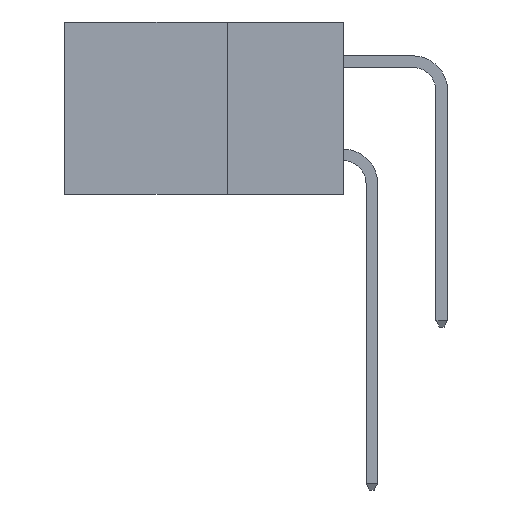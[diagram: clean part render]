
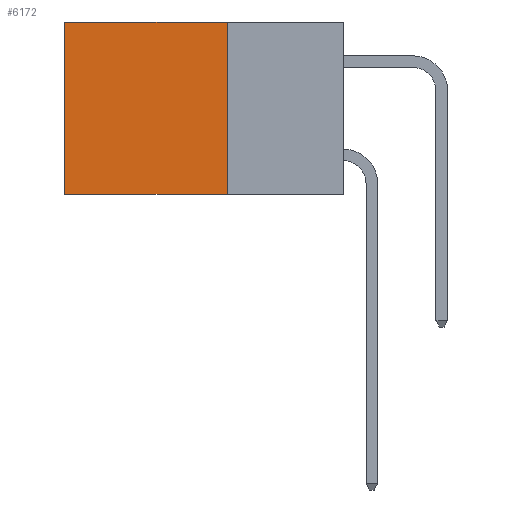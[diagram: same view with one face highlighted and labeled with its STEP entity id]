
A CAD part, left-side view. The second image highlights one B-rep face of the part: STEP entity #6172.
In plain terms, the highlighted planar face has unit normal (-1, 0, 0).
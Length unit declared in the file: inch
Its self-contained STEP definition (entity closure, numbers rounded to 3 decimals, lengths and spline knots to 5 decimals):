
#212 = DIRECTION ( 'NONE',  ( 0., 1., 0. ) ) ;
#258 = CARTESIAN_POINT ( 'NONE',  ( 0.2615, 0.25, 0. ) ) ;
#278 = VECTOR ( 'NONE', #212, 39.37008 ) ;
#1241 = CARTESIAN_POINT ( 'NONE',  ( 0.2615, 0.25, -0.37 ) ) ;
#1265 = DIRECTION ( 'NONE',  ( 0., 1., 0. ) ) ;
#1739 = CARTESIAN_POINT ( 'NONE',  ( 0.2615, 0.25, 0. ) ) ;
#3355 = VERTEX_POINT ( 'NONE', #7405 ) ;
#3881 = VECTOR ( 'NONE', #13143, 39.37008 ) ;
#4373 = VERTEX_POINT ( 'NONE', #7060 ) ;
#4594 = EDGE_CURVE ( 'NONE', #17309, #3355, #11534, .T. ) ;
#5127 = VECTOR ( 'NONE', #11169, 39.37008 ) ;
#5345 = VERTEX_POINT ( 'NONE', #12327 ) ;
#5991 = DIRECTION ( 'NONE',  ( 0., 0., -1. ) ) ;
#6032 = DIRECTION ( 'NONE',  ( 1., 0., 0. ) ) ;
#6057 = PLANE ( 'NONE',  #12001 ) ;
#6172 = ADVANCED_FACE ( 'NONE', ( #11684 ), #6057, .F. ) ;
#6360 = CARTESIAN_POINT ( 'NONE',  ( 0.2615, 0.25, -0.37 ) ) ;
#6794 = EDGE_CURVE ( 'NONE', #5345, #4373, #7202, .T. ) ;
#7060 = CARTESIAN_POINT ( 'NONE',  ( 0.2615, 0.6, -0.37 ) ) ;
#7202 = LINE ( 'NONE', #1241, #16959 ) ;
#7405 = CARTESIAN_POINT ( 'NONE',  ( 0.2615, 0.6, 0. ) ) ;
#7982 = EDGE_CURVE ( 'NONE', #3355, #4373, #16332, .T. ) ;
#8663 = ORIENTED_EDGE ( 'NONE', *, *, #7982, .T. ) ;
#9659 = ORIENTED_EDGE ( 'NONE', *, *, #11011, .F. ) ;
#11011 = EDGE_CURVE ( 'NONE', #17309, #5345, #11710, .T. ) ;
#11169 = DIRECTION ( 'NONE',  ( 0., 0., -1. ) ) ;
#11534 = LINE ( 'NONE', #258, #278 ) ;
#11684 = FACE_OUTER_BOUND ( 'NONE', #11731, .T. ) ;
#11710 = LINE ( 'NONE', #11935, #3881 ) ;
#11731 = EDGE_LOOP ( 'NONE', ( #8663, #15746, #9659, #12449 ) ) ;
#11935 = CARTESIAN_POINT ( 'NONE',  ( 0.2615, 0.25, -0.37 ) ) ;
#12001 = AXIS2_PLACEMENT_3D ( 'NONE', #6360, #6032, #5991 ) ;
#12327 = CARTESIAN_POINT ( 'NONE',  ( 0.2615, 0.25, -0.37 ) ) ;
#12449 = ORIENTED_EDGE ( 'NONE', *, *, #4594, .T. ) ;
#12486 = CARTESIAN_POINT ( 'NONE',  ( 0.2615, 0.6, -0.37 ) ) ;
#13143 = DIRECTION ( 'NONE',  ( 0., 0., -1. ) ) ;
#15746 = ORIENTED_EDGE ( 'NONE', *, *, #6794, .F. ) ;
#16332 = LINE ( 'NONE', #12486, #5127 ) ;
#16959 = VECTOR ( 'NONE', #1265, 39.37008 ) ;
#17309 = VERTEX_POINT ( 'NONE', #1739 ) ;
